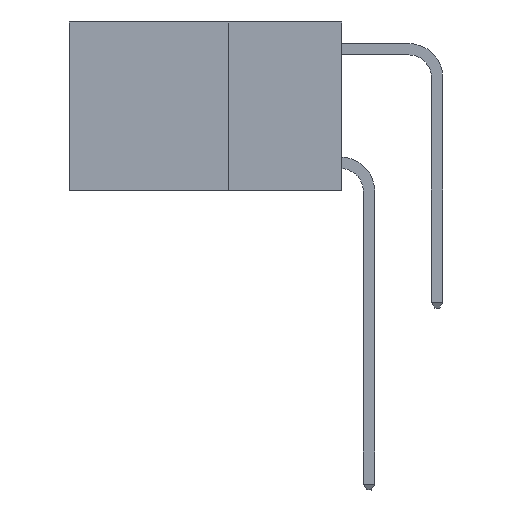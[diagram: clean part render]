
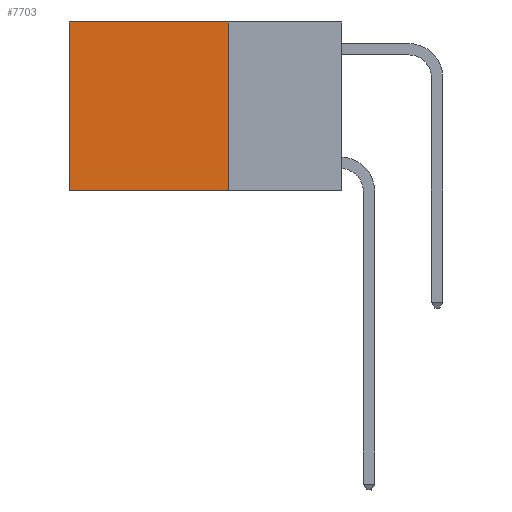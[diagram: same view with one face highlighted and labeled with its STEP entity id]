
A CAD part, left-side view. The second image highlights one B-rep face of the part: STEP entity #7703.
In plain terms, the highlighted planar face has unit normal (-1, 0, 0).
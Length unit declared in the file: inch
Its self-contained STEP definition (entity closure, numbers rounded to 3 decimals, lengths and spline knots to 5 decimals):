
#824 = DIRECTION ( 'NONE',  ( 1., 0., 0. ) ) ;
#1191 = ORIENTED_EDGE ( 'NONE', *, *, #14051, .F. ) ;
#1280 = ORIENTED_EDGE ( 'NONE', *, *, #1983, .F. ) ;
#1422 = LINE ( 'NONE', #16845, #5767 ) ;
#1471 = VERTEX_POINT ( 'NONE', #11904 ) ;
#1837 = LINE ( 'NONE', #20571, #11610 ) ;
#1983 = EDGE_CURVE ( 'NONE', #1471, #19656, #1422, .T. ) ;
#2244 = DIRECTION ( 'NONE',  ( 0., 0., -1. ) ) ;
#2786 = CARTESIAN_POINT ( 'NONE',  ( 0.2625, 0.25, 0. ) ) ;
#2965 = VECTOR ( 'NONE', #7650, 39.37008 ) ;
#3561 = FACE_OUTER_BOUND ( 'NONE', #7507, .T. ) ;
#5767 = VECTOR ( 'NONE', #2244, 39.37008 ) ;
#7507 = EDGE_LOOP ( 'NONE', ( #19766, #1191, #1280, #17079 ) ) ;
#7650 = DIRECTION ( 'NONE',  ( 0., 0., -1. ) ) ;
#7703 = ADVANCED_FACE ( 'NONE', ( #3561 ), #8188, .F. ) ;
#7897 = CARTESIAN_POINT ( 'NONE',  ( 0.2625, 0.6, 0. ) ) ;
#8188 = PLANE ( 'NONE',  #9964 ) ;
#8926 = EDGE_CURVE ( 'NONE', #9053, #18818, #11577, .T. ) ;
#9053 = VERTEX_POINT ( 'NONE', #7897 ) ;
#9770 = DIRECTION ( 'NONE',  ( 0., 1., 0. ) ) ;
#9872 = CARTESIAN_POINT ( 'NONE',  ( 0.2625, 0.25, -0.37 ) ) ;
#9964 = AXIS2_PLACEMENT_3D ( 'NONE', #15372, #824, #13636 ) ;
#11577 = LINE ( 'NONE', #18462, #2965 ) ;
#11610 = VECTOR ( 'NONE', #9770, 39.37008 ) ;
#11904 = CARTESIAN_POINT ( 'NONE',  ( 0.2625, 0.25, 0. ) ) ;
#13022 = EDGE_CURVE ( 'NONE', #1471, #9053, #18994, .T. ) ;
#13089 = VECTOR ( 'NONE', #13730, 39.37008 ) ;
#13636 = DIRECTION ( 'NONE',  ( 0., 0., -1. ) ) ;
#13730 = DIRECTION ( 'NONE',  ( 0., 1., 0. ) ) ;
#14051 = EDGE_CURVE ( 'NONE', #19656, #18818, #1837, .T. ) ;
#15372 = CARTESIAN_POINT ( 'NONE',  ( 0.2625, 0.25, 0. ) ) ;
#16845 = CARTESIAN_POINT ( 'NONE',  ( 0.2625, 0.25, 0. ) ) ;
#17079 = ORIENTED_EDGE ( 'NONE', *, *, #13022, .T. ) ;
#18462 = CARTESIAN_POINT ( 'NONE',  ( 0.2625, 0.6, 0. ) ) ;
#18818 = VERTEX_POINT ( 'NONE', #22878 ) ;
#18994 = LINE ( 'NONE', #2786, #13089 ) ;
#19656 = VERTEX_POINT ( 'NONE', #9872 ) ;
#19766 = ORIENTED_EDGE ( 'NONE', *, *, #8926, .T. ) ;
#20571 = CARTESIAN_POINT ( 'NONE',  ( 0.2625, 0.25, -0.37 ) ) ;
#22878 = CARTESIAN_POINT ( 'NONE',  ( 0.2625, 0.6, -0.37 ) ) ;
